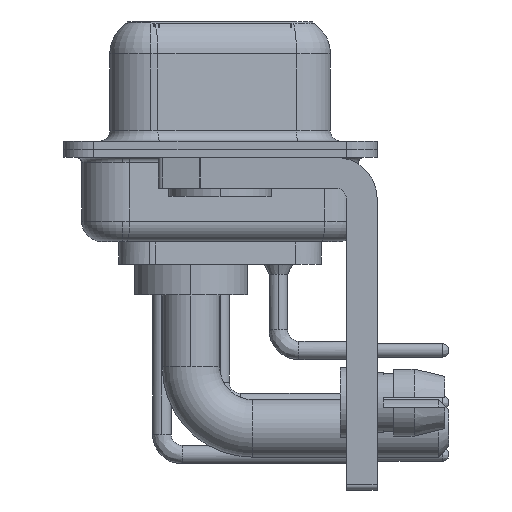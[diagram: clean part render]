
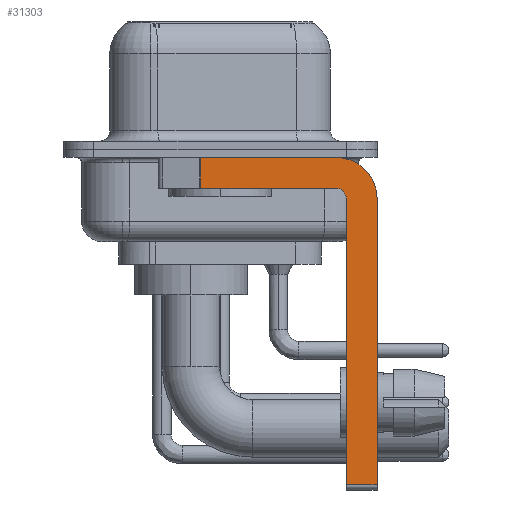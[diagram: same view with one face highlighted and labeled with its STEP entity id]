
A CAD part, left-side view. The second image highlights one B-rep face of the part: STEP entity #31303.
In plain terms, the highlighted planar face has unit normal (-1, 0, 0).
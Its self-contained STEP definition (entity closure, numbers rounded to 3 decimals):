
#241 = VECTOR ( 'NONE', #6993, 1000. ) ;
#601 = CARTESIAN_POINT ( 'NONE',  ( -2.9, -5.65, -1.9 ) ) ;
#750 = AXIS2_PLACEMENT_3D ( 'NONE', #17906, #3437, #27680 ) ;
#768 = VERTEX_POINT ( 'NONE', #30039 ) ;
#1492 = EDGE_LOOP ( 'NONE', ( #31031, #26359, #20196, #20924, #7047, #17439, #21871, #21174 ) ) ;
#2060 = VECTOR ( 'NONE', #30299, 1000. ) ;
#2637 = CARTESIAN_POINT ( 'NONE',  ( -2.9, 0.978, -0.4 ) ) ;
#3275 = CARTESIAN_POINT ( 'NONE',  ( -2.9, 0.978, -1.9 ) ) ;
#3339 = VERTEX_POINT ( 'NONE', #26261 ) ;
#3361 = CARTESIAN_POINT ( 'NONE',  ( -2.9, -6.15, -16.6 ) ) ;
#3437 = DIRECTION ( 'NONE',  ( 1., 0., 0. ) ) ;
#3675 = DIRECTION ( 'NONE',  ( 0., -1., 0. ) ) ;
#4274 = FACE_OUTER_BOUND ( 'NONE', #1492, .T. ) ;
#4339 = CIRCLE ( 'NONE', #750, 2. ) ;
#5633 = DIRECTION ( 'NONE',  ( 0., 0., 1. ) ) ;
#5704 = LINE ( 'NONE', #3275, #24317 ) ;
#5846 = CARTESIAN_POINT ( 'NONE',  ( -2.9, -5.65, -2.4 ) ) ;
#5946 = CIRCLE ( 'NONE', #7993, 0.5 ) ;
#6248 = VECTOR ( 'NONE', #3675, 1000. ) ;
#6654 = EDGE_CURVE ( 'NONE', #27059, #18653, #15236, .T. ) ;
#6993 = DIRECTION ( 'NONE',  ( 0., -1., 0. ) ) ;
#7047 = ORIENTED_EDGE ( 'NONE', *, *, #28699, .F. ) ;
#7087 = VECTOR ( 'NONE', #5633, 1000. ) ;
#7531 = CARTESIAN_POINT ( 'NONE',  ( -2.9, -7.65, -2.4 ) ) ;
#7993 = AXIS2_PLACEMENT_3D ( 'NONE', #5846, #15157, #13094 ) ;
#8761 = VERTEX_POINT ( 'NONE', #29442 ) ;
#9004 = EDGE_CURVE ( 'NONE', #23210, #18653, #5704, .T. ) ;
#9147 = EDGE_CURVE ( 'NONE', #23210, #8761, #28972, .T. ) ;
#9411 = CARTESIAN_POINT ( 'NONE',  ( -2.9, 3., -0.4 ) ) ;
#10050 = AXIS2_PLACEMENT_3D ( 'NONE', #21464, #31242, #19051 ) ;
#11083 = EDGE_CURVE ( 'NONE', #19948, #27059, #5946, .T. ) ;
#12971 = VERTEX_POINT ( 'NONE', #30348 ) ;
#13094 = DIRECTION ( 'NONE',  ( 0., 0., 1. ) ) ;
#13102 = DIRECTION ( 'NONE',  ( 0., 0., -1. ) ) ;
#14718 = PLANE ( 'NONE',  #10050 ) ;
#15157 = DIRECTION ( 'NONE',  ( -1., 0., 0. ) ) ;
#15236 = LINE ( 'NONE', #601, #2060 ) ;
#15581 = LINE ( 'NONE', #3361, #7087 ) ;
#16423 = CARTESIAN_POINT ( 'NONE',  ( -2.9, 0.978, -1.9 ) ) ;
#17320 = DIRECTION ( 'NONE',  ( 0., 0., -1. ) ) ;
#17439 = ORIENTED_EDGE ( 'NONE', *, *, #17835, .T. ) ;
#17835 = EDGE_CURVE ( 'NONE', #12971, #3339, #26141, .T. ) ;
#17906 = CARTESIAN_POINT ( 'NONE',  ( -2.9, -5.65, -2.4 ) ) ;
#18653 = VERTEX_POINT ( 'NONE', #16423 ) ;
#19051 = DIRECTION ( 'NONE',  ( 0., 0., -1. ) ) ;
#19407 = EDGE_CURVE ( 'NONE', #768, #3339, #29504, .T. ) ;
#19948 = VERTEX_POINT ( 'NONE', #29788 ) ;
#20196 = ORIENTED_EDGE ( 'NONE', *, *, #6654, .F. ) ;
#20924 = ORIENTED_EDGE ( 'NONE', *, *, #11083, .F. ) ;
#21174 = ORIENTED_EDGE ( 'NONE', *, *, #26003, .F. ) ;
#21464 = CARTESIAN_POINT ( 'NONE',  ( -2.9, -5.65, -2.4 ) ) ;
#21871 = ORIENTED_EDGE ( 'NONE', *, *, #19407, .F. ) ;
#22010 = VECTOR ( 'NONE', #17320, 1000. ) ;
#23210 = VERTEX_POINT ( 'NONE', #2637 ) ;
#23611 = CARTESIAN_POINT ( 'NONE',  ( -2.9, -5.65, -1.9 ) ) ;
#24317 = VECTOR ( 'NONE', #13102, 1000. ) ;
#26003 = EDGE_CURVE ( 'NONE', #8761, #768, #4339, .T. ) ;
#26141 = LINE ( 'NONE', #28382, #6248 ) ;
#26261 = CARTESIAN_POINT ( 'NONE',  ( -2.9, -7.65, -16.35 ) ) ;
#26359 = ORIENTED_EDGE ( 'NONE', *, *, #9004, .T. ) ;
#27059 = VERTEX_POINT ( 'NONE', #23611 ) ;
#27680 = DIRECTION ( 'NONE',  ( 0., 0., -1. ) ) ;
#28382 = CARTESIAN_POINT ( 'NONE',  ( -2.9, -5.65, -16.35 ) ) ;
#28699 = EDGE_CURVE ( 'NONE', #12971, #19948, #15581, .T. ) ;
#28972 = LINE ( 'NONE', #9411, #241 ) ;
#29442 = CARTESIAN_POINT ( 'NONE',  ( -2.9, -5.65, -0.4 ) ) ;
#29504 = LINE ( 'NONE', #7531, #22010 ) ;
#29788 = CARTESIAN_POINT ( 'NONE',  ( -2.9, -6.15, -2.4 ) ) ;
#30039 = CARTESIAN_POINT ( 'NONE',  ( -2.9, -7.65, -2.4 ) ) ;
#30299 = DIRECTION ( 'NONE',  ( 0., 1., 0. ) ) ;
#30348 = CARTESIAN_POINT ( 'NONE',  ( -2.9, -6.15, -16.35 ) ) ;
#31031 = ORIENTED_EDGE ( 'NONE', *, *, #9147, .F. ) ;
#31242 = DIRECTION ( 'NONE',  ( 1., 0., 0. ) ) ;
#31303 = ADVANCED_FACE ( 'NONE', ( #4274 ), #14718, .F. ) ;
